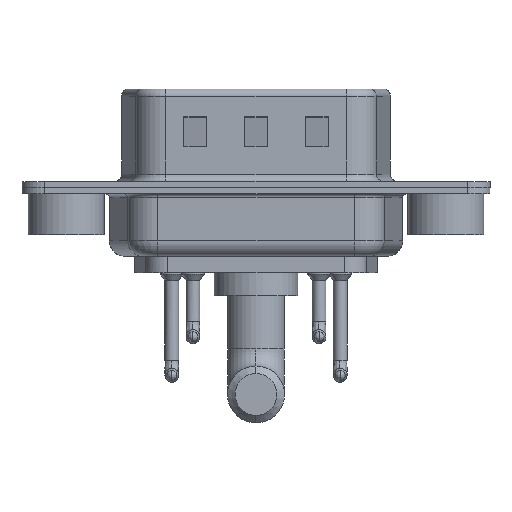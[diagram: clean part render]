
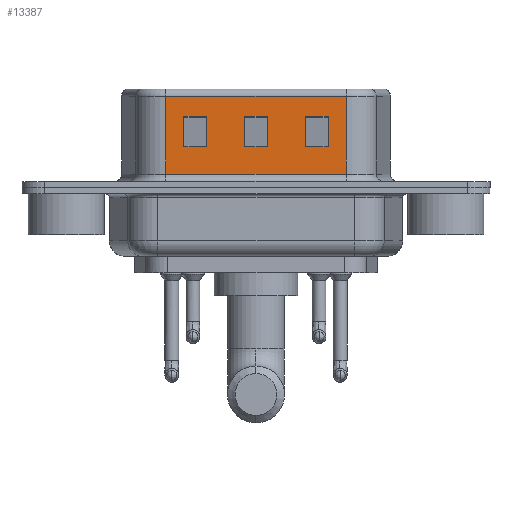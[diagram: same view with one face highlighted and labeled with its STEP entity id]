
A CAD part, front view. The second image highlights one B-rep face of the part: STEP entity #13387.
In plain terms, the highlighted planar face has unit normal (0, -1, 0).
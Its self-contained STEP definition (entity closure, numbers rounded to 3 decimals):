
#317 = DIRECTION ( 'NONE',  ( 0., 0., -1. ) ) ;
#531 = DIRECTION ( 'NONE',  ( 0., 0., -1. ) ) ;
#600 = EDGE_CURVE ( 'NONE', #10324, #2400, #8933, .T. ) ;
#791 = ORIENTED_EDGE ( 'NONE', *, *, #16804, .T. ) ;
#873 = CARTESIAN_POINT ( 'NONE',  ( 7.75, -4.55, 4.705 ) ) ;
#926 = CARTESIAN_POINT ( 'NONE',  ( 15.75, -4.55, 2.705 ) ) ;
#1123 = LINE ( 'NONE', #8674, #14263 ) ;
#1356 = DIRECTION ( 'NONE',  ( 0., 0., -1. ) ) ;
#1473 = LINE ( 'NONE', #8925, #11827 ) ;
#1696 = CARTESIAN_POINT ( 'NONE',  ( 13.25, -4.55, 4.705 ) ) ;
#2012 = DIRECTION ( 'NONE',  ( -1., 0., 0. ) ) ;
#2118 = ORIENTED_EDGE ( 'NONE', *, *, #4088, .T. ) ;
#2225 = DIRECTION ( 'NONE',  ( 0., 0., 1. ) ) ;
#2356 = CARTESIAN_POINT ( 'NONE',  ( 9.25, -4.55, 4.705 ) ) ;
#2400 = VERTEX_POINT ( 'NONE', #926 ) ;
#2566 = DIRECTION ( 'NONE',  ( 0., 0., 1. ) ) ;
#2626 = ORIENTED_EDGE ( 'NONE', *, *, #11952, .T. ) ;
#2664 = VERTEX_POINT ( 'NONE', #17689 ) ;
#2678 = ORIENTED_EDGE ( 'NONE', *, *, #19093, .T. ) ;
#2796 = LINE ( 'NONE', #5620, #16479 ) ;
#2908 = DIRECTION ( 'NONE',  ( -1., 0., 0. ) ) ;
#3335 = VECTOR ( 'NONE', #2908, 1000. ) ;
#3582 = VERTEX_POINT ( 'NONE', #7695 ) ;
#3631 = ORIENTED_EDGE ( 'NONE', *, *, #17947, .T. ) ;
#3640 = LINE ( 'NONE', #13878, #10203 ) ;
#3773 = CARTESIAN_POINT ( 'NONE',  ( 11.75, -4.55, 6.52 ) ) ;
#3905 = CARTESIAN_POINT ( 'NONE',  ( 11.75, -4.55, 4.705 ) ) ;
#4088 = EDGE_CURVE ( 'NONE', #12624, #15784, #1473, .T. ) ;
#4122 = ORIENTED_EDGE ( 'NONE', *, *, #17188, .T. ) ;
#4373 = AXIS2_PLACEMENT_3D ( 'NONE', #18486, #17196, #2012 ) ;
#4576 = ORIENTED_EDGE ( 'NONE', *, *, #9523, .T. ) ;
#4629 = CARTESIAN_POINT ( 'NONE',  ( 15.75, -4.55, 4.705 ) ) ;
#4677 = VERTEX_POINT ( 'NONE', #15217 ) ;
#4835 = VERTEX_POINT ( 'NONE', #10039 ) ;
#5145 = LINE ( 'NONE', #3773, #10588 ) ;
#5302 = EDGE_LOOP ( 'NONE', ( #15956, #791, #16724, #14201 ) ) ;
#5401 = VECTOR ( 'NONE', #10495, 1000. ) ;
#5423 = EDGE_CURVE ( 'NONE', #12555, #2664, #13842, .T. ) ;
#5428 = DIRECTION ( 'NONE',  ( -1., 0., 0. ) ) ;
#5461 = CARTESIAN_POINT ( 'NONE',  ( 17.25, -4.55, 6.52 ) ) ;
#5517 = VERTEX_POINT ( 'NONE', #873 ) ;
#5620 = CARTESIAN_POINT ( 'NONE',  ( 14.451, -4.55, 2.705 ) ) ;
#5624 = EDGE_CURVE ( 'NONE', #7952, #10324, #18900, .T. ) ;
#5657 = EDGE_LOOP ( 'NONE', ( #9964, #2626, #4122, #10443 ) ) ;
#5821 = LINE ( 'NONE', #11818, #5896 ) ;
#5896 = VECTOR ( 'NONE', #17911, 1000. ) ;
#6140 = CARTESIAN_POINT ( 'NONE',  ( 22.451, -4.55, 4.705 ) ) ;
#6564 = EDGE_CURVE ( 'NONE', #4835, #3582, #12748, .T. ) ;
#6681 = LINE ( 'NONE', #6140, #7148 ) ;
#7062 = CARTESIAN_POINT ( 'NONE',  ( 18.451, -4.55, 0.9 ) ) ;
#7148 = VECTOR ( 'NONE', #16535, 1000. ) ;
#7242 = ORIENTED_EDGE ( 'NONE', *, *, #16960, .T. ) ;
#7250 = LINE ( 'NONE', #19208, #7806 ) ;
#7568 = DIRECTION ( 'NONE',  ( 1., 0., 0. ) ) ;
#7650 = EDGE_CURVE ( 'NONE', #18060, #3582, #13412, .T. ) ;
#7695 = CARTESIAN_POINT ( 'NONE',  ( 18.451, -4.55, 0.9 ) ) ;
#7806 = VECTOR ( 'NONE', #19301, 1000. ) ;
#7952 = VERTEX_POINT ( 'NONE', #18761 ) ;
#8000 = EDGE_CURVE ( 'NONE', #5517, #12555, #16029, .T. ) ;
#8006 = EDGE_LOOP ( 'NONE', ( #2118, #4576, #3631, #13922 ) ) ;
#8183 = FACE_OUTER_BOUND ( 'NONE', #5657, .T. ) ;
#8582 = CARTESIAN_POINT ( 'NONE',  ( 18.451, -4.55, 6.02 ) ) ;
#8674 = CARTESIAN_POINT ( 'NONE',  ( 15.75, -4.55, 6.52 ) ) ;
#8678 = LINE ( 'NONE', #19061, #3335 ) ;
#8731 = CARTESIAN_POINT ( 'NONE',  ( 22.451, -4.55, 2.705 ) ) ;
#8925 = CARTESIAN_POINT ( 'NONE',  ( 18.451, -4.55, 4.705 ) ) ;
#8933 = LINE ( 'NONE', #8731, #5401 ) ;
#9229 = VERTEX_POINT ( 'NONE', #4629 ) ;
#9523 = EDGE_CURVE ( 'NONE', #15784, #10494, #7250, .T. ) ;
#9546 = VERTEX_POINT ( 'NONE', #13020 ) ;
#9964 = ORIENTED_EDGE ( 'NONE', *, *, #7650, .F. ) ;
#10001 = DIRECTION ( 'NONE',  ( 1., 0., 0. ) ) ;
#10039 = CARTESIAN_POINT ( 'NONE',  ( 6.549, -4.55, 0.9 ) ) ;
#10203 = VECTOR ( 'NONE', #531, 1000. ) ;
#10324 = VERTEX_POINT ( 'NONE', #13888 ) ;
#10443 = ORIENTED_EDGE ( 'NONE', *, *, #6564, .T. ) ;
#10494 = VERTEX_POINT ( 'NONE', #13397 ) ;
#10495 = DIRECTION ( 'NONE',  ( -1., 0., 0. ) ) ;
#10588 = VECTOR ( 'NONE', #2225, 1000. ) ;
#10691 = VECTOR ( 'NONE', #11362, 1000. ) ;
#10936 = FACE_BOUND ( 'NONE', #13596, .T. ) ;
#11362 = DIRECTION ( 'NONE',  ( 0., 0., -1. ) ) ;
#11642 = VECTOR ( 'NONE', #10001, 1000. ) ;
#11647 = ORIENTED_EDGE ( 'NONE', *, *, #5624, .T. ) ;
#11678 = CARTESIAN_POINT ( 'NONE',  ( 7.75, -4.55, 6.52 ) ) ;
#11818 = CARTESIAN_POINT ( 'NONE',  ( 18.451, -4.55, 6.02 ) ) ;
#11827 = VECTOR ( 'NONE', #7568, 1000. ) ;
#11952 = EDGE_CURVE ( 'NONE', #18060, #4677, #5821, .T. ) ;
#12024 = ORIENTED_EDGE ( 'NONE', *, *, #600, .T. ) ;
#12068 = CARTESIAN_POINT ( 'NONE',  ( 9.25, -4.55, 6.52 ) ) ;
#12555 = VERTEX_POINT ( 'NONE', #2356 ) ;
#12624 = VERTEX_POINT ( 'NONE', #3905 ) ;
#12748 = LINE ( 'NONE', #7062, #11642 ) ;
#12979 = CARTESIAN_POINT ( 'NONE',  ( 14.451, -4.55, 4.705 ) ) ;
#13020 = CARTESIAN_POINT ( 'NONE',  ( 7.75, -4.55, 2.705 ) ) ;
#13087 = DIRECTION ( 'NONE',  ( 0., 0., 1. ) ) ;
#13387 = ADVANCED_FACE ( 'NONE', ( #17100, #10936, #15451, #8183 ), #18756, .F. ) ;
#13397 = CARTESIAN_POINT ( 'NONE',  ( 13.25, -4.55, 2.705 ) ) ;
#13412 = LINE ( 'NONE', #14791, #15109 ) ;
#13596 = EDGE_LOOP ( 'NONE', ( #11647, #12024, #7242, #2678 ) ) ;
#13842 = LINE ( 'NONE', #12068, #15668 ) ;
#13878 = CARTESIAN_POINT ( 'NONE',  ( 6.549, -4.55, 6.52 ) ) ;
#13888 = CARTESIAN_POINT ( 'NONE',  ( 17.25, -4.55, 2.705 ) ) ;
#13922 = ORIENTED_EDGE ( 'NONE', *, *, #18729, .T. ) ;
#14072 = EDGE_CURVE ( 'NONE', #9546, #5517, #17456, .T. ) ;
#14201 = ORIENTED_EDGE ( 'NONE', *, *, #8000, .T. ) ;
#14263 = VECTOR ( 'NONE', #13087, 1000. ) ;
#14337 = CARTESIAN_POINT ( 'NONE',  ( 11.75, -4.55, 2.705 ) ) ;
#14791 = CARTESIAN_POINT ( 'NONE',  ( 18.451, -4.55, 6.52 ) ) ;
#15109 = VECTOR ( 'NONE', #1356, 1000. ) ;
#15217 = CARTESIAN_POINT ( 'NONE',  ( 6.549, -4.55, 6.02 ) ) ;
#15451 = FACE_BOUND ( 'NONE', #8006, .T. ) ;
#15668 = VECTOR ( 'NONE', #317, 1000. ) ;
#15784 = VERTEX_POINT ( 'NONE', #1696 ) ;
#15956 = ORIENTED_EDGE ( 'NONE', *, *, #5423, .T. ) ;
#16029 = LINE ( 'NONE', #12979, #17909 ) ;
#16479 = VECTOR ( 'NONE', #5428, 1000. ) ;
#16535 = DIRECTION ( 'NONE',  ( 1., 0., 0. ) ) ;
#16641 = VECTOR ( 'NONE', #2566, 1000. ) ;
#16724 = ORIENTED_EDGE ( 'NONE', *, *, #14072, .T. ) ;
#16804 = EDGE_CURVE ( 'NONE', #2664, #9546, #2796, .T. ) ;
#16960 = EDGE_CURVE ( 'NONE', #2400, #9229, #1123, .T. ) ;
#17100 = FACE_BOUND ( 'NONE', #5302, .T. ) ;
#17188 = EDGE_CURVE ( 'NONE', #4677, #4835, #3640, .T. ) ;
#17196 = DIRECTION ( 'NONE',  ( 0., 1., 0. ) ) ;
#17456 = LINE ( 'NONE', #11678, #16641 ) ;
#17689 = CARTESIAN_POINT ( 'NONE',  ( 9.25, -4.55, 2.705 ) ) ;
#17909 = VECTOR ( 'NONE', #18949, 1000. ) ;
#17911 = DIRECTION ( 'NONE',  ( -1., 0., 0. ) ) ;
#17947 = EDGE_CURVE ( 'NONE', #10494, #18502, #8678, .T. ) ;
#18060 = VERTEX_POINT ( 'NONE', #8582 ) ;
#18486 = CARTESIAN_POINT ( 'NONE',  ( 18.451, -4.55, 6.52 ) ) ;
#18502 = VERTEX_POINT ( 'NONE', #14337 ) ;
#18729 = EDGE_CURVE ( 'NONE', #18502, #12624, #5145, .T. ) ;
#18756 = PLANE ( 'NONE',  #4373 ) ;
#18761 = CARTESIAN_POINT ( 'NONE',  ( 17.25, -4.55, 4.705 ) ) ;
#18900 = LINE ( 'NONE', #5461, #10691 ) ;
#18949 = DIRECTION ( 'NONE',  ( 1., 0., 0. ) ) ;
#19061 = CARTESIAN_POINT ( 'NONE',  ( 18.451, -4.55, 2.705 ) ) ;
#19093 = EDGE_CURVE ( 'NONE', #9229, #7952, #6681, .T. ) ;
#19208 = CARTESIAN_POINT ( 'NONE',  ( 13.25, -4.55, 6.52 ) ) ;
#19301 = DIRECTION ( 'NONE',  ( 0., 0., -1. ) ) ;
